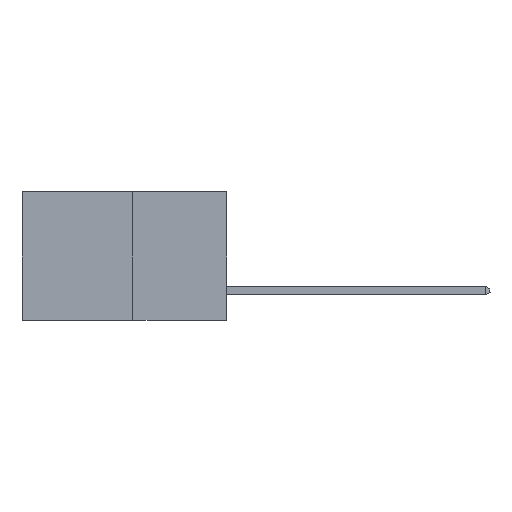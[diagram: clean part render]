
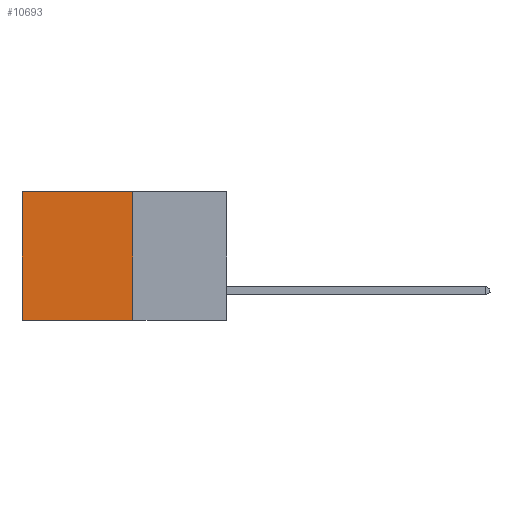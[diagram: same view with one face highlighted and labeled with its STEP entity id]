
A CAD part, left-side view. The second image highlights one B-rep face of the part: STEP entity #10693.
In plain terms, the highlighted planar face has unit normal (-1, 0, 0).
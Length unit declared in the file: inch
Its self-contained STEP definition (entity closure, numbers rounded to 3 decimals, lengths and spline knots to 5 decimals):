
#624 = CARTESIAN_POINT ( 'NONE',  ( 0.277, 0.27, 0. ) ) ;
#826 = CARTESIAN_POINT ( 'NONE',  ( 0.277, 0.59, 0. ) ) ;
#858 = VECTOR ( 'NONE', #14273, 39.37008 ) ;
#1138 = DIRECTION ( 'NONE',  ( 0., 1., 0. ) ) ;
#1187 = CARTESIAN_POINT ( 'NONE',  ( 0.277, 0.59, -0.37 ) ) ;
#1327 = AXIS2_PLACEMENT_3D ( 'NONE', #4260, #12921, #5506 ) ;
#2374 = CARTESIAN_POINT ( 'NONE',  ( 0.277, 0.27, -0.37 ) ) ;
#3129 = DIRECTION ( 'NONE',  ( 0., 1., 0. ) ) ;
#3166 = CARTESIAN_POINT ( 'NONE',  ( 0.277, 0.27, -0.37 ) ) ;
#3942 = FACE_OUTER_BOUND ( 'NONE', #8111, .T. ) ;
#4260 = CARTESIAN_POINT ( 'NONE',  ( 0.277, 0.27, -0.37 ) ) ;
#4772 = LINE ( 'NONE', #2374, #14268 ) ;
#5328 = EDGE_CURVE ( 'NONE', #10703, #11324, #7429, .T. ) ;
#5506 = DIRECTION ( 'NONE',  ( 0., 0., -1. ) ) ;
#5735 = CARTESIAN_POINT ( 'NONE',  ( 0.277, 0.27, -0.37 ) ) ;
#6510 = EDGE_CURVE ( 'NONE', #10703, #11986, #15144, .T. ) ;
#7106 = CARTESIAN_POINT ( 'NONE',  ( 0.277, 0.59, -0.37 ) ) ;
#7429 = LINE ( 'NONE', #3166, #858 ) ;
#8111 = EDGE_LOOP ( 'NONE', ( #9230, #12371, #8745, #8902 ) ) ;
#8224 = VECTOR ( 'NONE', #13304, 39.37008 ) ;
#8745 = ORIENTED_EDGE ( 'NONE', *, *, #5328, .F. ) ;
#8902 = ORIENTED_EDGE ( 'NONE', *, *, #6510, .T. ) ;
#9230 = ORIENTED_EDGE ( 'NONE', *, *, #14924, .T. ) ;
#9784 = VERTEX_POINT ( 'NONE', #1187 ) ;
#10693 = ADVANCED_FACE ( 'NONE', ( #3942 ), #15337, .F. ) ;
#10703 = VERTEX_POINT ( 'NONE', #11687 ) ;
#11324 = VERTEX_POINT ( 'NONE', #5735 ) ;
#11687 = CARTESIAN_POINT ( 'NONE',  ( 0.277, 0.27, 0. ) ) ;
#11986 = VERTEX_POINT ( 'NONE', #826 ) ;
#12253 = VECTOR ( 'NONE', #3129, 39.37008 ) ;
#12371 = ORIENTED_EDGE ( 'NONE', *, *, #13843, .F. ) ;
#12921 = DIRECTION ( 'NONE',  ( 1., 0., 0. ) ) ;
#13304 = DIRECTION ( 'NONE',  ( 0., 0., -1. ) ) ;
#13843 = EDGE_CURVE ( 'NONE', #11324, #9784, #4772, .T. ) ;
#14268 = VECTOR ( 'NONE', #1138, 39.37008 ) ;
#14273 = DIRECTION ( 'NONE',  ( 0., 0., -1. ) ) ;
#14924 = EDGE_CURVE ( 'NONE', #11986, #9784, #15554, .T. ) ;
#15144 = LINE ( 'NONE', #624, #12253 ) ;
#15337 = PLANE ( 'NONE',  #1327 ) ;
#15554 = LINE ( 'NONE', #7106, #8224 ) ;
